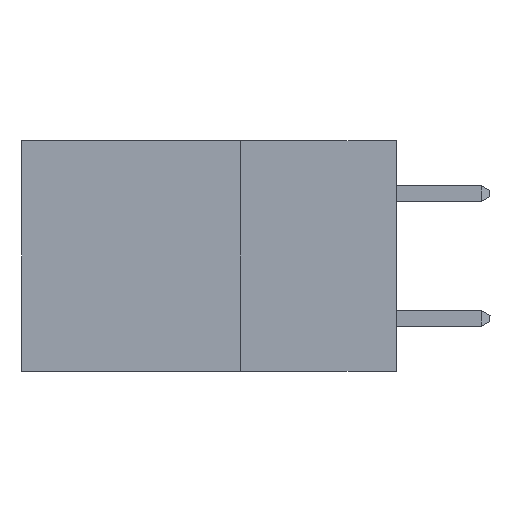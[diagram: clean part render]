
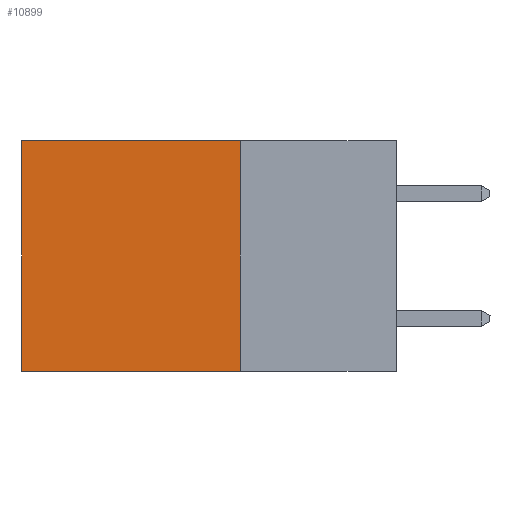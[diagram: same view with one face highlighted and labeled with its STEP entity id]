
A CAD part, left-side view. The second image highlights one B-rep face of the part: STEP entity #10899.
In plain terms, the highlighted planar face has unit normal (-1, 0, 0).
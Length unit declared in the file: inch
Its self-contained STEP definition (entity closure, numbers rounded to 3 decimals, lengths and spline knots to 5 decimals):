
#843 = AXIS2_PLACEMENT_3D ( 'NONE', #8701, #26319, #21376 ) ;
#1349 = VERTEX_POINT ( 'NONE', #28165 ) ;
#1511 = PLANE ( 'NONE',  #843 ) ;
#2638 = LINE ( 'NONE', #3902, #32127 ) ;
#2914 = EDGE_CURVE ( 'NONE', #7098, #1349, #10263, .T. ) ;
#2993 = CARTESIAN_POINT ( 'NONE',  ( 0.298, 0.25, 0. ) ) ;
#3902 = CARTESIAN_POINT ( 'NONE',  ( 0.298, 0.6, 0. ) ) ;
#5203 = VECTOR ( 'NONE', #6575, 39.37008 ) ;
#5527 = DIRECTION ( 'NONE',  ( 0., 0., -1. ) ) ;
#5904 = LINE ( 'NONE', #2993, #32256 ) ;
#6575 = DIRECTION ( 'NONE',  ( 0., 1., 0. ) ) ;
#7098 = VERTEX_POINT ( 'NONE', #13209 ) ;
#8339 = DIRECTION ( 'NONE',  ( 0., 1., 0. ) ) ;
#8654 = VERTEX_POINT ( 'NONE', #22588 ) ;
#8701 = CARTESIAN_POINT ( 'NONE',  ( 0.298, 0.25, 0. ) ) ;
#8854 = DIRECTION ( 'NONE',  ( 0., 0., -1. ) ) ;
#10263 = LINE ( 'NONE', #24661, #5203 ) ;
#10899 = ADVANCED_FACE ( 'NONE', ( #14439 ), #1511, .F. ) ;
#13209 = CARTESIAN_POINT ( 'NONE',  ( 0.298, 0.25, -0.37 ) ) ;
#14439 = FACE_OUTER_BOUND ( 'NONE', #29184, .T. ) ;
#14641 = EDGE_CURVE ( 'NONE', #8654, #7098, #5904, .T. ) ;
#15203 = VECTOR ( 'NONE', #8339, 39.37008 ) ;
#21376 = DIRECTION ( 'NONE',  ( 0., 0., -1. ) ) ;
#21830 = EDGE_CURVE ( 'NONE', #24221, #1349, #2638, .T. ) ;
#22588 = CARTESIAN_POINT ( 'NONE',  ( 0.298, 0.25, 0. ) ) ;
#23054 = CARTESIAN_POINT ( 'NONE',  ( 0.298, 0.6, 0. ) ) ;
#23146 = EDGE_CURVE ( 'NONE', #8654, #24221, #25106, .T. ) ;
#23670 = CARTESIAN_POINT ( 'NONE',  ( 0.298, 0.25, 0. ) ) ;
#24221 = VERTEX_POINT ( 'NONE', #23054 ) ;
#24661 = CARTESIAN_POINT ( 'NONE',  ( 0.298, 0.25, -0.37 ) ) ;
#25037 = ORIENTED_EDGE ( 'NONE', *, *, #23146, .T. ) ;
#25106 = LINE ( 'NONE', #23670, #15203 ) ;
#26319 = DIRECTION ( 'NONE',  ( 1., 0., 0. ) ) ;
#28165 = CARTESIAN_POINT ( 'NONE',  ( 0.298, 0.6, -0.37 ) ) ;
#29184 = EDGE_LOOP ( 'NONE', ( #29572, #30010, #31493, #25037 ) ) ;
#29572 = ORIENTED_EDGE ( 'NONE', *, *, #21830, .T. ) ;
#30010 = ORIENTED_EDGE ( 'NONE', *, *, #2914, .F. ) ;
#31493 = ORIENTED_EDGE ( 'NONE', *, *, #14641, .F. ) ;
#32127 = VECTOR ( 'NONE', #8854, 39.37008 ) ;
#32256 = VECTOR ( 'NONE', #5527, 39.37008 ) ;
